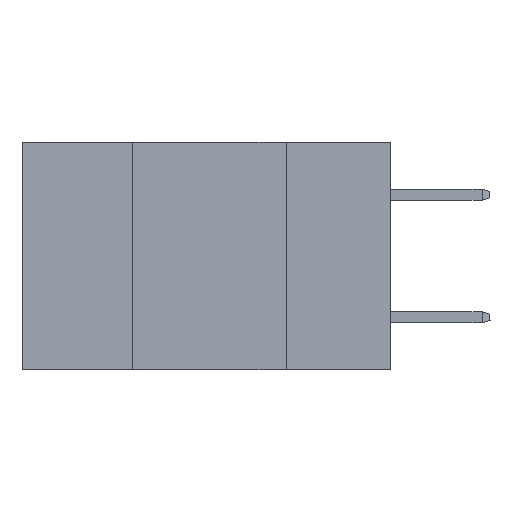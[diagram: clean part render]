
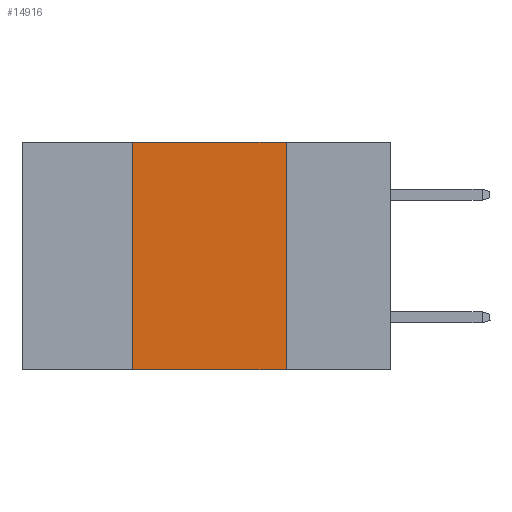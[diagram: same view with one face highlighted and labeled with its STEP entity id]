
A CAD part, left-side view. The second image highlights one B-rep face of the part: STEP entity #14916.
In plain terms, the highlighted planar face has unit normal (-1, 0, 0).
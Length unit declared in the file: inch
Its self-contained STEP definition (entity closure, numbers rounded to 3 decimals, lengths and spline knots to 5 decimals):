
#250 = CARTESIAN_POINT ( 'NONE',  ( 0., 0.6, -0.37 ) ) ;
#264 = CARTESIAN_POINT ( 'NONE',  ( 0., 0.6, 0. ) ) ;
#778 = VECTOR ( 'NONE', #1679, 39.37008 ) ;
#797 = VERTEX_POINT ( 'NONE', #9200 ) ;
#1283 = ORIENTED_EDGE ( 'NONE', *, *, #10016, .T. ) ;
#1408 = CARTESIAN_POINT ( 'NONE',  ( 0., 0.17, -0.37 ) ) ;
#1435 = PLANE ( 'NONE',  #7621 ) ;
#1513 = DIRECTION ( 'NONE',  ( 0., -1., 0. ) ) ;
#1679 = DIRECTION ( 'NONE',  ( 0., -1., 0. ) ) ;
#2122 = CARTESIAN_POINT ( 'NONE',  ( 0., 0.17, 0. ) ) ;
#2132 = VERTEX_POINT ( 'NONE', #14741 ) ;
#2252 = ORIENTED_EDGE ( 'NONE', *, *, #15854, .F. ) ;
#2290 = DIRECTION ( 'NONE',  ( 0., 0., -1. ) ) ;
#4201 = LINE ( 'NONE', #14397, #778 ) ;
#4246 = LINE ( 'NONE', #7245, #13074 ) ;
#5096 = EDGE_CURVE ( 'NONE', #2132, #9712, #14692, .T. ) ;
#6798 = CARTESIAN_POINT ( 'NONE',  ( 0., 0.42, 0. ) ) ;
#7245 = CARTESIAN_POINT ( 'NONE',  ( 0., 0.42, 0. ) ) ;
#7621 = AXIS2_PLACEMENT_3D ( 'NONE', #264, #15539, #13125 ) ;
#7632 = FACE_OUTER_BOUND ( 'NONE', #11892, .T. ) ;
#8087 = EDGE_CURVE ( 'NONE', #10435, #2132, #4201, .T. ) ;
#8293 = LINE ( 'NONE', #250, #10245 ) ;
#8580 = DIRECTION ( 'NONE',  ( 0., 0., 1. ) ) ;
#9200 = CARTESIAN_POINT ( 'NONE',  ( 0., 0.42, -0.37 ) ) ;
#9712 = VERTEX_POINT ( 'NONE', #1408 ) ;
#10016 = EDGE_CURVE ( 'NONE', #797, #9712, #8293, .T. ) ;
#10245 = VECTOR ( 'NONE', #1513, 39.37008 ) ;
#10435 = VERTEX_POINT ( 'NONE', #6798 ) ;
#11784 = ORIENTED_EDGE ( 'NONE', *, *, #8087, .F. ) ;
#11892 = EDGE_LOOP ( 'NONE', ( #15308, #11784, #2252, #1283 ) ) ;
#12942 = VECTOR ( 'NONE', #2290, 39.37008 ) ;
#13074 = VECTOR ( 'NONE', #8580, 39.37008 ) ;
#13125 = DIRECTION ( 'NONE',  ( 0., 0., -1. ) ) ;
#14397 = CARTESIAN_POINT ( 'NONE',  ( 0., 0.6, 0. ) ) ;
#14692 = LINE ( 'NONE', #2122, #12942 ) ;
#14741 = CARTESIAN_POINT ( 'NONE',  ( 0., 0.17, 0. ) ) ;
#14916 = ADVANCED_FACE ( 'NONE', ( #7632 ), #1435, .F. ) ;
#15308 = ORIENTED_EDGE ( 'NONE', *, *, #5096, .F. ) ;
#15539 = DIRECTION ( 'NONE',  ( 1., 0., 0. ) ) ;
#15854 = EDGE_CURVE ( 'NONE', #797, #10435, #4246, .T. ) ;
